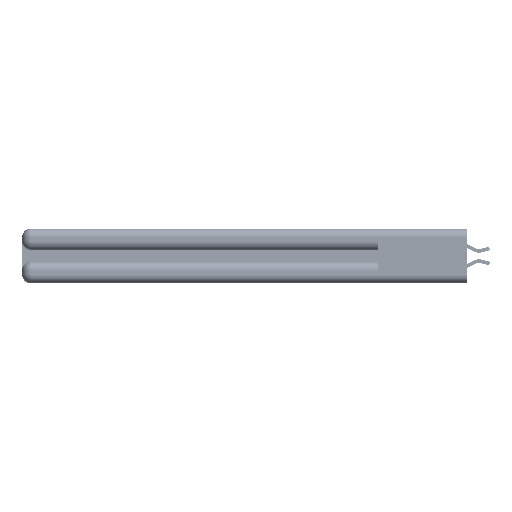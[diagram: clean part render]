
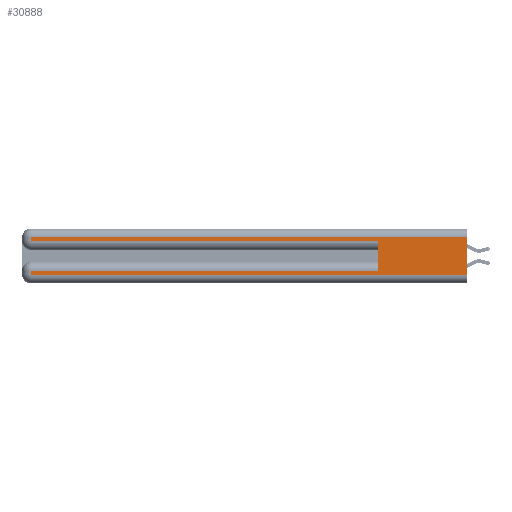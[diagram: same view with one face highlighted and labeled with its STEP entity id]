
A CAD part, left-side view. The second image highlights one B-rep face of the part: STEP entity #30888.
In plain terms, the highlighted planar face has unit normal (-1, 0, 0).
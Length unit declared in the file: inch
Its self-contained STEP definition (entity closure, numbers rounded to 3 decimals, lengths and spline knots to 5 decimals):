
#1697 = VERTEX_POINT ( 'NONE', #50871 ) ;
#1703 = ORIENTED_EDGE ( 'NONE', *, *, #55071, .T. ) ;
#2100 = EDGE_CURVE ( 'NONE', #1697, #55669, #43376, .T. ) ;
#2179 = CARTESIAN_POINT ( 'NONE',  ( 0., 0., 0.285 ) ) ;
#2529 = VERTEX_POINT ( 'NONE', #9040 ) ;
#3103 = EDGE_LOOP ( 'NONE', ( #17897, #53831, #1703, #35583, #35810, #16359, #45159, #52568 ) ) ;
#3218 = CARTESIAN_POINT ( 'NONE',  ( 0., 0., 0.31 ) ) ;
#4809 = EDGE_CURVE ( 'NONE', #54656, #43318, #21278, .T. ) ;
#4973 = CARTESIAN_POINT ( 'NONE',  ( 0., 2.94, 0.085 ) ) ;
#6666 = DIRECTION ( 'NONE',  ( 0., -1., 0. ) ) ;
#9040 = CARTESIAN_POINT ( 'NONE',  ( 0., 2.94, 0.06 ) ) ;
#13859 = DIRECTION ( 'NONE',  ( 0., -1., 0. ) ) ;
#15062 = CARTESIAN_POINT ( 'NONE',  ( 0., 0., 0.06 ) ) ;
#15724 = DIRECTION ( 'NONE',  ( 0., 0., -1. ) ) ;
#16359 = ORIENTED_EDGE ( 'NONE', *, *, #23269, .T. ) ;
#16967 = PLANE ( 'NONE',  #56019 ) ;
#17897 = ORIENTED_EDGE ( 'NONE', *, *, #32633, .F. ) ;
#17968 = CARTESIAN_POINT ( 'NONE',  ( 0., 0., 0.31 ) ) ;
#20359 = VECTOR ( 'NONE', #50880, 39.37008 ) ;
#21278 = LINE ( 'NONE', #3218, #41731 ) ;
#21753 = EDGE_CURVE ( 'NONE', #2529, #32655, #22226, .T. ) ;
#22226 = LINE ( 'NONE', #44371, #33862 ) ;
#23269 = EDGE_CURVE ( 'NONE', #1697, #33984, #52800, .T. ) ;
#25743 = CARTESIAN_POINT ( 'NONE',  ( 0., 0., 0.37 ) ) ;
#26597 = VERTEX_POINT ( 'NONE', #53220 ) ;
#26816 = LINE ( 'NONE', #45189, #48599 ) ;
#28473 = VECTOR ( 'NONE', #15724, 39.37008 ) ;
#29217 = CARTESIAN_POINT ( 'NONE',  ( 0., 2.94, 0.37 ) ) ;
#29862 = CARTESIAN_POINT ( 'NONE',  ( 0., 2.94, 0.31 ) ) ;
#30138 = DIRECTION ( 'NONE',  ( 0., 0., -1. ) ) ;
#30446 = EDGE_CURVE ( 'NONE', #26597, #55669, #53575, .T. ) ;
#30529 = LINE ( 'NONE', #29217, #20359 ) ;
#30888 = ADVANCED_FACE ( 'NONE', ( #42024 ), #16967, .F. ) ;
#31642 = DIRECTION ( 'NONE',  ( 0., 0., 1. ) ) ;
#32419 = DIRECTION ( 'NONE',  ( 0., 1., 0. ) ) ;
#32633 = EDGE_CURVE ( 'NONE', #54656, #32655, #26816, .T. ) ;
#32655 = VERTEX_POINT ( 'NONE', #15062 ) ;
#33180 = VECTOR ( 'NONE', #31642, 39.37008 ) ;
#33862 = VECTOR ( 'NONE', #13859, 39.37008 ) ;
#33984 = VERTEX_POINT ( 'NONE', #4973 ) ;
#35583 = ORIENTED_EDGE ( 'NONE', *, *, #30446, .T. ) ;
#35810 = ORIENTED_EDGE ( 'NONE', *, *, #2100, .F. ) ;
#37507 = CARTESIAN_POINT ( 'NONE',  ( 0., 2.94, 0.37 ) ) ;
#38305 = DIRECTION ( 'NONE',  ( 0., 1., 0. ) ) ;
#38575 = VECTOR ( 'NONE', #32419, 39.37008 ) ;
#38720 = LINE ( 'NONE', #37507, #28473 ) ;
#41731 = VECTOR ( 'NONE', #38305, 39.37008 ) ;
#42024 = FACE_OUTER_BOUND ( 'NONE', #3103, .T. ) ;
#42507 = CARTESIAN_POINT ( 'NONE',  ( 0., 0.6, 0.285 ) ) ;
#43318 = VERTEX_POINT ( 'NONE', #29862 ) ;
#43376 = LINE ( 'NONE', #53274, #33180 ) ;
#44371 = CARTESIAN_POINT ( 'NONE',  ( 0., 0., 0.06 ) ) ;
#45159 = ORIENTED_EDGE ( 'NONE', *, *, #56189, .T. ) ;
#45189 = CARTESIAN_POINT ( 'NONE',  ( 0., 0., 0.37 ) ) ;
#48599 = VECTOR ( 'NONE', #49549, 39.37008 ) ;
#49549 = DIRECTION ( 'NONE',  ( 0., 0., -1. ) ) ;
#50871 = CARTESIAN_POINT ( 'NONE',  ( 0., 0.6, 0.085 ) ) ;
#50880 = DIRECTION ( 'NONE',  ( 0., 0., -1. ) ) ;
#52235 = VECTOR ( 'NONE', #6666, 39.37008 ) ;
#52568 = ORIENTED_EDGE ( 'NONE', *, *, #21753, .T. ) ;
#52800 = LINE ( 'NONE', #54052, #38575 ) ;
#53220 = CARTESIAN_POINT ( 'NONE',  ( 0., 2.94, 0.285 ) ) ;
#53274 = CARTESIAN_POINT ( 'NONE',  ( 0., 0.6, 0.145 ) ) ;
#53575 = LINE ( 'NONE', #2179, #52235 ) ;
#53831 = ORIENTED_EDGE ( 'NONE', *, *, #4809, .T. ) ;
#54052 = CARTESIAN_POINT ( 'NONE',  ( 0., 0., 0.085 ) ) ;
#54656 = VERTEX_POINT ( 'NONE', #17968 ) ;
#55071 = EDGE_CURVE ( 'NONE', #43318, #26597, #30529, .T. ) ;
#55669 = VERTEX_POINT ( 'NONE', #42507 ) ;
#56019 = AXIS2_PLACEMENT_3D ( 'NONE', #25743, #56120, #30138 ) ;
#56120 = DIRECTION ( 'NONE',  ( 1., 0., 0. ) ) ;
#56189 = EDGE_CURVE ( 'NONE', #33984, #2529, #38720, .T. ) ;
